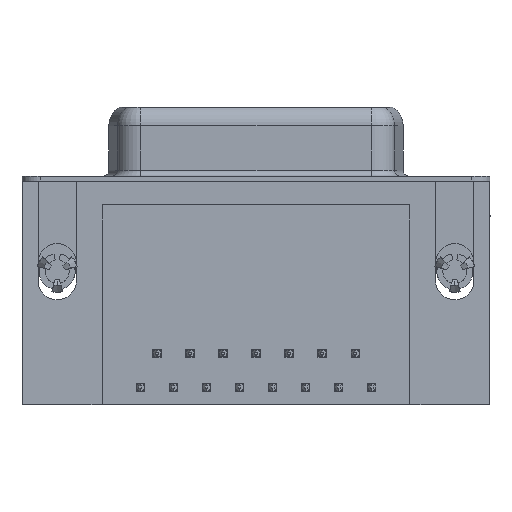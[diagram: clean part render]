
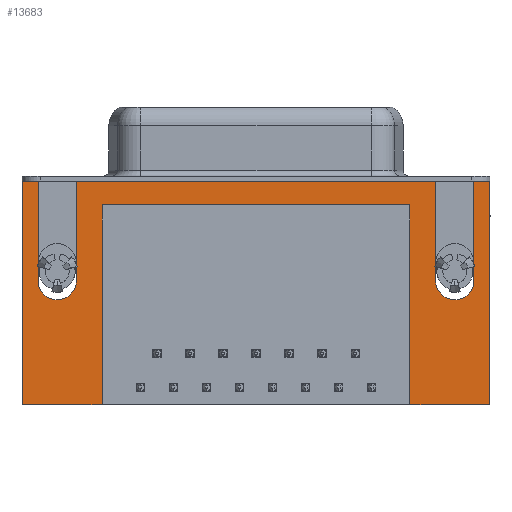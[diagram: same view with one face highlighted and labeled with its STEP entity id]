
A CAD part, front view. The second image highlights one B-rep face of the part: STEP entity #13683.
In plain terms, the highlighted planar face has unit normal (0, -1, 0).
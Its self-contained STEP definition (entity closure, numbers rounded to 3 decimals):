
#865 = DIRECTION ( 'NONE',  ( 0., 0., -1. ) ) ;
#908 = VERTEX_POINT ( 'NONE', #4057 ) ;
#1297 = EDGE_CURVE ( 'NONE', #11580, #8076, #24453, .T. ) ;
#1323 = DIRECTION ( 'NONE',  ( 0., -1., 0. ) ) ;
#1600 = LINE ( 'NONE', #21166, #23234 ) ;
#1700 = DIRECTION ( 'NONE',  ( 0., 0., 1. ) ) ;
#1828 = LINE ( 'NONE', #10200, #27846 ) ;
#2403 = EDGE_CURVE ( 'NONE', #11902, #11668, #13779, .T. ) ;
#2554 = ORIENTED_EDGE ( 'NONE', *, *, #2786, .F. ) ;
#2786 = EDGE_CURVE ( 'NONE', #17312, #908, #17779, .T. ) ;
#2815 = EDGE_CURVE ( 'NONE', #3921, #26353, #12064, .T. ) ;
#2930 = LINE ( 'NONE', #6760, #8704 ) ;
#3066 = VECTOR ( 'NONE', #26375, 1000. ) ;
#3092 = VERTEX_POINT ( 'NONE', #12153 ) ;
#3477 = EDGE_CURVE ( 'NONE', #908, #26549, #27864, .T. ) ;
#3560 = CARTESIAN_POINT ( 'NONE',  ( 36.255, -6.275, -18.76 ) ) ;
#3777 = VECTOR ( 'NONE', #22975, 1000. ) ;
#3921 = VERTEX_POINT ( 'NONE', #3560 ) ;
#3947 = CARTESIAN_POINT ( 'NONE',  ( 36.255, -6.275, 0. ) ) ;
#4057 = CARTESIAN_POINT ( 'NONE',  ( 34.92, -6.275, 0. ) ) ;
#4165 = CARTESIAN_POINT ( 'NONE',  ( 1.6, -6.275, 0. ) ) ;
#4883 = VECTOR ( 'NONE', #16193, 1000. ) ;
#4938 = VERTEX_POINT ( 'NONE', #17229 ) ;
#5131 = CARTESIAN_POINT ( 'NONE',  ( -2.935, -6.275, -2.5 ) ) ;
#5324 = ORIENTED_EDGE ( 'NONE', *, *, #8905, .F. ) ;
#5398 = CARTESIAN_POINT ( 'NONE',  ( 33.32, -6.275, -8.35 ) ) ;
#6098 = DIRECTION ( 'NONE',  ( 0., 0., 1. ) ) ;
#6293 = VECTOR ( 'NONE', #6098, 1000. ) ;
#6408 = ORIENTED_EDGE ( 'NONE', *, *, #27730, .F. ) ;
#6597 = VERTEX_POINT ( 'NONE', #7276 ) ;
#6760 = CARTESIAN_POINT ( 'NONE',  ( 36.255, -6.275, -2.5 ) ) ;
#7276 = CARTESIAN_POINT ( 'NONE',  ( 3.765, -6.275, -2. ) ) ;
#7292 = VERTEX_POINT ( 'NONE', #23972 ) ;
#7319 = EDGE_LOOP ( 'NONE', ( #2554, #11618, #15318, #27740, #5324, #9776, #13911, #13812, #16702, #24550, #25059, #15040, #6408, #9254, #26576, #27078 ) ) ;
#7326 = DIRECTION ( 'NONE',  ( 0., 0., 1. ) ) ;
#7583 = DIRECTION ( 'NONE',  ( -1., 0., 0. ) ) ;
#8076 = VERTEX_POINT ( 'NONE', #19250 ) ;
#8081 = CARTESIAN_POINT ( 'NONE',  ( 34.92, -6.275, 0. ) ) ;
#8615 = VECTOR ( 'NONE', #7326, 1000. ) ;
#8704 = VECTOR ( 'NONE', #19676, 1000. ) ;
#8709 = VECTOR ( 'NONE', #15695, 1000. ) ;
#8905 = EDGE_CURVE ( 'NONE', #3092, #9605, #15722, .T. ) ;
#8944 = EDGE_CURVE ( 'NONE', #7292, #11560, #14374, .T. ) ;
#9087 = FACE_OUTER_BOUND ( 'NONE', #7319, .T. ) ;
#9249 = VERTEX_POINT ( 'NONE', #11589 ) ;
#9254 = ORIENTED_EDGE ( 'NONE', *, *, #2815, .F. ) ;
#9605 = VERTEX_POINT ( 'NONE', #4165 ) ;
#9662 = VECTOR ( 'NONE', #865, 1000. ) ;
#9776 = ORIENTED_EDGE ( 'NONE', *, *, #11487, .F. ) ;
#9786 = CARTESIAN_POINT ( 'NONE',  ( 31.72, -6.275, 0. ) ) ;
#10071 = CARTESIAN_POINT ( 'NONE',  ( 3.765, -6.275, -2. ) ) ;
#10200 = CARTESIAN_POINT ( 'NONE',  ( -2.935, -6.275, 0. ) ) ;
#10525 = AXIS2_PLACEMENT_3D ( 'NONE', #5398, #20501, #7583 ) ;
#10541 = EDGE_CURVE ( 'NONE', #11560, #11902, #13904, .T. ) ;
#10727 = CARTESIAN_POINT ( 'NONE',  ( 0., -6.275, -8.35 ) ) ;
#11487 = EDGE_CURVE ( 'NONE', #11668, #3092, #23621, .T. ) ;
#11560 = VERTEX_POINT ( 'NONE', #24874 ) ;
#11580 = VERTEX_POINT ( 'NONE', #9786 ) ;
#11589 = CARTESIAN_POINT ( 'NONE',  ( 3.765, -6.275, -18.76 ) ) ;
#11618 = ORIENTED_EDGE ( 'NONE', *, *, #16517, .F. ) ;
#11668 = VERTEX_POINT ( 'NONE', #25058 ) ;
#11902 = VERTEX_POINT ( 'NONE', #25894 ) ;
#12064 = LINE ( 'NONE', #23194, #22166 ) ;
#12126 = PLANE ( 'NONE',  #18968 ) ;
#12153 = CARTESIAN_POINT ( 'NONE',  ( 1.6, -6.275, -8.35 ) ) ;
#12679 = DIRECTION ( 'NONE',  ( 0., 0., -1. ) ) ;
#12915 = DIRECTION ( 'NONE',  ( 1., 0., 0. ) ) ;
#13417 = CIRCLE ( 'NONE', #10525, 1.6 ) ;
#13477 = CARTESIAN_POINT ( 'NONE',  ( -2.935, -6.275, 0. ) ) ;
#13678 = CARTESIAN_POINT ( 'NONE',  ( 1.6, -6.275, 0. ) ) ;
#13683 = ADVANCED_FACE ( 'NONE', ( #9087 ), #12126, .T. ) ;
#13779 = LINE ( 'NONE', #21526, #8709 ) ;
#13812 = ORIENTED_EDGE ( 'NONE', *, *, #10541, .F. ) ;
#13901 = CARTESIAN_POINT ( 'NONE',  ( 29.555, -6.275, -18.76 ) ) ;
#13904 = LINE ( 'NONE', #13477, #3066 ) ;
#13911 = ORIENTED_EDGE ( 'NONE', *, *, #2403, .F. ) ;
#14374 = LINE ( 'NONE', #5131, #8615 ) ;
#15040 = ORIENTED_EDGE ( 'NONE', *, *, #23799, .F. ) ;
#15303 = LINE ( 'NONE', #10071, #3777 ) ;
#15318 = ORIENTED_EDGE ( 'NONE', *, *, #1297, .F. ) ;
#15695 = DIRECTION ( 'NONE',  ( 0., 0., -1. ) ) ;
#15722 = LINE ( 'NONE', #13678, #26506 ) ;
#16003 = CARTESIAN_POINT ( 'NONE',  ( 3.765, -6.275, -2. ) ) ;
#16193 = DIRECTION ( 'NONE',  ( 1., 0., 0. ) ) ;
#16457 = DIRECTION ( 'NONE',  ( 0., 0., -1. ) ) ;
#16517 = EDGE_CURVE ( 'NONE', #8076, #17312, #13417, .T. ) ;
#16693 = DIRECTION ( 'NONE',  ( -1., 0., 0. ) ) ;
#16702 = ORIENTED_EDGE ( 'NONE', *, *, #8944, .F. ) ;
#17080 = EDGE_CURVE ( 'NONE', #9605, #11580, #1828, .T. ) ;
#17229 = CARTESIAN_POINT ( 'NONE',  ( 29.555, -6.275, -2. ) ) ;
#17312 = VERTEX_POINT ( 'NONE', #21882 ) ;
#17779 = LINE ( 'NONE', #8081, #6293 ) ;
#17804 = CARTESIAN_POINT ( 'NONE',  ( 36.255, -6.275, -18.76 ) ) ;
#17894 = DIRECTION ( 'NONE',  ( 0., 0., 1. ) ) ;
#18117 = VECTOR ( 'NONE', #19952, 1000. ) ;
#18707 = VECTOR ( 'NONE', #12679, 1000. ) ;
#18963 = EDGE_CURVE ( 'NONE', #3921, #26549, #2930, .T. ) ;
#18968 = AXIS2_PLACEMENT_3D ( 'NONE', #27184, #1323, #16457 ) ;
#19044 = EDGE_CURVE ( 'NONE', #9249, #7292, #24546, .T. ) ;
#19250 = CARTESIAN_POINT ( 'NONE',  ( 31.72, -6.275, -8.35 ) ) ;
#19676 = DIRECTION ( 'NONE',  ( 0., 0., 1. ) ) ;
#19952 = DIRECTION ( 'NONE',  ( -1., 0., 0. ) ) ;
#20501 = DIRECTION ( 'NONE',  ( 0., -1., 0. ) ) ;
#20702 = EDGE_CURVE ( 'NONE', #6597, #9249, #26882, .T. ) ;
#21166 = CARTESIAN_POINT ( 'NONE',  ( 29.555, -6.275, -2. ) ) ;
#21526 = CARTESIAN_POINT ( 'NONE',  ( -1.6, -6.275, 0. ) ) ;
#21882 = CARTESIAN_POINT ( 'NONE',  ( 34.92, -6.275, -8.35 ) ) ;
#22166 = VECTOR ( 'NONE', #16693, 1000. ) ;
#22975 = DIRECTION ( 'NONE',  ( -1., 0., 0. ) ) ;
#23117 = DIRECTION ( 'NONE',  ( 1., 0., 0. ) ) ;
#23194 = CARTESIAN_POINT ( 'NONE',  ( 36.255, -6.275, -18.76 ) ) ;
#23234 = VECTOR ( 'NONE', #1700, 1000. ) ;
#23621 = CIRCLE ( 'NONE', #24719, 1.6 ) ;
#23799 = EDGE_CURVE ( 'NONE', #4938, #6597, #15303, .T. ) ;
#23972 = CARTESIAN_POINT ( 'NONE',  ( -2.935, -6.275, -18.76 ) ) ;
#24453 = LINE ( 'NONE', #25131, #18707 ) ;
#24546 = LINE ( 'NONE', #17804, #18117 ) ;
#24550 = ORIENTED_EDGE ( 'NONE', *, *, #19044, .F. ) ;
#24719 = AXIS2_PLACEMENT_3D ( 'NONE', #10727, #25819, #12915 ) ;
#24874 = CARTESIAN_POINT ( 'NONE',  ( -2.935, -6.275, 0. ) ) ;
#25058 = CARTESIAN_POINT ( 'NONE',  ( -1.6, -6.275, -8.35 ) ) ;
#25059 = ORIENTED_EDGE ( 'NONE', *, *, #20702, .F. ) ;
#25131 = CARTESIAN_POINT ( 'NONE',  ( 31.72, -6.275, 0. ) ) ;
#25819 = DIRECTION ( 'NONE',  ( 0., -1., 0. ) ) ;
#25894 = CARTESIAN_POINT ( 'NONE',  ( -1.6, -6.275, 0. ) ) ;
#26353 = VERTEX_POINT ( 'NONE', #13901 ) ;
#26375 = DIRECTION ( 'NONE',  ( 1., 0., 0. ) ) ;
#26506 = VECTOR ( 'NONE', #17894, 1000. ) ;
#26549 = VERTEX_POINT ( 'NONE', #3947 ) ;
#26576 = ORIENTED_EDGE ( 'NONE', *, *, #18963, .T. ) ;
#26882 = LINE ( 'NONE', #16003, #9662 ) ;
#26941 = CARTESIAN_POINT ( 'NONE',  ( -2.935, -6.275, 0. ) ) ;
#27078 = ORIENTED_EDGE ( 'NONE', *, *, #3477, .F. ) ;
#27184 = CARTESIAN_POINT ( 'NONE',  ( -2.935, -6.275, -2.5 ) ) ;
#27730 = EDGE_CURVE ( 'NONE', #26353, #4938, #1600, .T. ) ;
#27740 = ORIENTED_EDGE ( 'NONE', *, *, #17080, .F. ) ;
#27846 = VECTOR ( 'NONE', #23117, 1000. ) ;
#27864 = LINE ( 'NONE', #26941, #4883 ) ;
